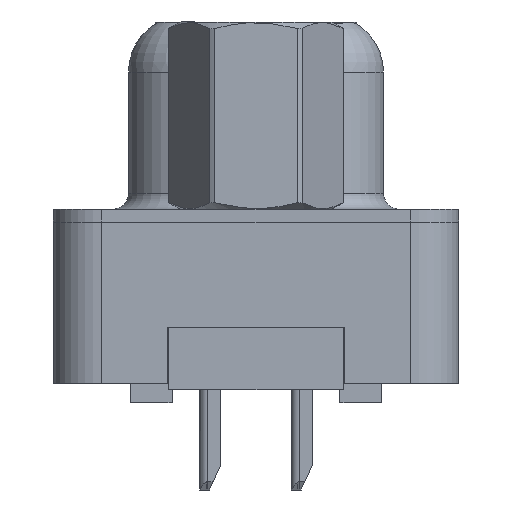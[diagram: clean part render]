
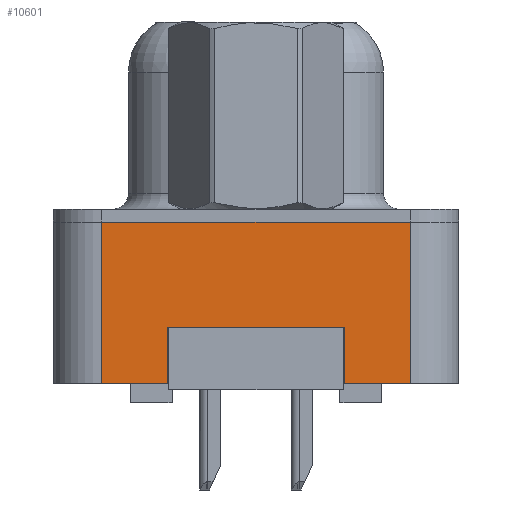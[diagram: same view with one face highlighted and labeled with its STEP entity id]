
A CAD part, left-side view. The second image highlights one B-rep face of the part: STEP entity #10601.
In plain terms, the highlighted planar face has unit normal (-1, 0, 0).
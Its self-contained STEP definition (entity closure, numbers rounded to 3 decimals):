
#666 = LINE ( 'NONE', #20459, #3838 ) ;
#901 = CARTESIAN_POINT ( 'NONE',  ( -2.995, -2.75, -3.25 ) ) ;
#1080 = CARTESIAN_POINT ( 'NONE',  ( -2.995, -4.775, 0. ) ) ;
#1109 = VECTOR ( 'NONE', #14346, 1000. ) ;
#1584 = CARTESIAN_POINT ( 'NONE',  ( -2.995, -4.775, -5. ) ) ;
#1613 = LINE ( 'NONE', #11330, #8405 ) ;
#1839 = CARTESIAN_POINT ( 'NONE',  ( -2.995, 4.775, -5. ) ) ;
#3038 = VECTOR ( 'NONE', #20800, 1000. ) ;
#3346 = DIRECTION ( 'NONE',  ( 0., -1., 0. ) ) ;
#3684 = VERTEX_POINT ( 'NONE', #19237 ) ;
#3803 = VERTEX_POINT ( 'NONE', #18210 ) ;
#3838 = VECTOR ( 'NONE', #20339, 1000. ) ;
#4428 = EDGE_LOOP ( 'NONE', ( #9128, #5966, #21010, #17127, #9668, #17199, #22677, #19614 ) ) ;
#4459 = DIRECTION ( 'NONE',  ( 0., -1., 0. ) ) ;
#4594 = LINE ( 'NONE', #16162, #1109 ) ;
#4720 = VERTEX_POINT ( 'NONE', #9482 ) ;
#5484 = DIRECTION ( 'NONE',  ( -1., 0., 0. ) ) ;
#5966 = ORIENTED_EDGE ( 'NONE', *, *, #12718, .T. ) ;
#6107 = CARTESIAN_POINT ( 'NONE',  ( -2.995, -4.775, -5. ) ) ;
#6797 = VECTOR ( 'NONE', #4459, 1000. ) ;
#6803 = LINE ( 'NONE', #14538, #17442 ) ;
#7143 = PLANE ( 'NONE',  #8353 ) ;
#7261 = DIRECTION ( 'NONE',  ( 0., 0., 1. ) ) ;
#7532 = EDGE_CURVE ( 'NONE', #18362, #4720, #9463, .T. ) ;
#8353 = AXIS2_PLACEMENT_3D ( 'NONE', #23114, #5484, #18991 ) ;
#8405 = VECTOR ( 'NONE', #12860, 1000. ) ;
#9128 = ORIENTED_EDGE ( 'NONE', *, *, #10941, .T. ) ;
#9463 = LINE ( 'NONE', #17236, #3038 ) ;
#9482 = CARTESIAN_POINT ( 'NONE',  ( -2.995, 4.775, 0. ) ) ;
#9668 = ORIENTED_EDGE ( 'NONE', *, *, #7532, .F. ) ;
#10601 = ADVANCED_FACE ( 'NONE', ( #11198 ), #7143, .T. ) ;
#10941 = EDGE_CURVE ( 'NONE', #20710, #23076, #4594, .T. ) ;
#11198 = FACE_OUTER_BOUND ( 'NONE', #4428, .T. ) ;
#11208 = LINE ( 'NONE', #19000, #21288 ) ;
#11330 = CARTESIAN_POINT ( 'NONE',  ( -2.995, -4.775, -5. ) ) ;
#12036 = EDGE_CURVE ( 'NONE', #18362, #3803, #1613, .T. ) ;
#12489 = VERTEX_POINT ( 'NONE', #1080 ) ;
#12718 = EDGE_CURVE ( 'NONE', #23076, #3684, #17304, .T. ) ;
#12860 = DIRECTION ( 'NONE',  ( 0., -1., 0. ) ) ;
#14346 = DIRECTION ( 'NONE',  ( 0., 0., -1. ) ) ;
#14538 = CARTESIAN_POINT ( 'NONE',  ( -2.995, 2.75, -3.25 ) ) ;
#15100 = EDGE_CURVE ( 'NONE', #20710, #24050, #6803, .T. ) ;
#16162 = CARTESIAN_POINT ( 'NONE',  ( -2.995, -2.75, -3.25 ) ) ;
#16941 = CARTESIAN_POINT ( 'NONE',  ( -2.995, -2.75, -5. ) ) ;
#17127 = ORIENTED_EDGE ( 'NONE', *, *, #18225, .F. ) ;
#17199 = ORIENTED_EDGE ( 'NONE', *, *, #12036, .T. ) ;
#17236 = CARTESIAN_POINT ( 'NONE',  ( -2.995, 4.775, -5. ) ) ;
#17304 = LINE ( 'NONE', #6107, #6797 ) ;
#17442 = VECTOR ( 'NONE', #22290, 1000. ) ;
#18210 = CARTESIAN_POINT ( 'NONE',  ( -2.995, 2.75, -5. ) ) ;
#18225 = EDGE_CURVE ( 'NONE', #4720, #12489, #11208, .T. ) ;
#18362 = VERTEX_POINT ( 'NONE', #1839 ) ;
#18991 = DIRECTION ( 'NONE',  ( 0., 0., 1. ) ) ;
#19000 = CARTESIAN_POINT ( 'NONE',  ( -2.995, -4.775, 0. ) ) ;
#19237 = CARTESIAN_POINT ( 'NONE',  ( -2.995, -4.775, -5. ) ) ;
#19614 = ORIENTED_EDGE ( 'NONE', *, *, #15100, .F. ) ;
#20085 = EDGE_CURVE ( 'NONE', #24050, #3803, #666, .T. ) ;
#20339 = DIRECTION ( 'NONE',  ( 0., 0., -1. ) ) ;
#20459 = CARTESIAN_POINT ( 'NONE',  ( -2.995, 2.75, -3.25 ) ) ;
#20710 = VERTEX_POINT ( 'NONE', #901 ) ;
#20800 = DIRECTION ( 'NONE',  ( 0., 0., 1. ) ) ;
#21010 = ORIENTED_EDGE ( 'NONE', *, *, #21666, .T. ) ;
#21288 = VECTOR ( 'NONE', #3346, 1000. ) ;
#21666 = EDGE_CURVE ( 'NONE', #3684, #12489, #24769, .T. ) ;
#21731 = VECTOR ( 'NONE', #7261, 1000. ) ;
#22290 = DIRECTION ( 'NONE',  ( 0., 1., 0. ) ) ;
#22677 = ORIENTED_EDGE ( 'NONE', *, *, #20085, .F. ) ;
#23076 = VERTEX_POINT ( 'NONE', #16941 ) ;
#23114 = CARTESIAN_POINT ( 'NONE',  ( -2.995, -4.775, -5. ) ) ;
#23250 = CARTESIAN_POINT ( 'NONE',  ( -2.995, 2.75, -3.25 ) ) ;
#24050 = VERTEX_POINT ( 'NONE', #23250 ) ;
#24769 = LINE ( 'NONE', #1584, #21731 ) ;
